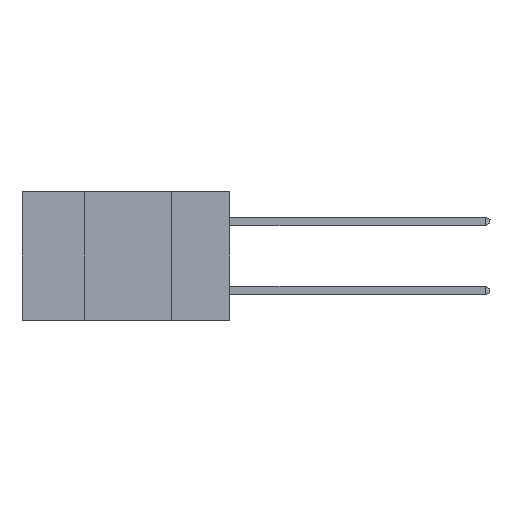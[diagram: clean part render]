
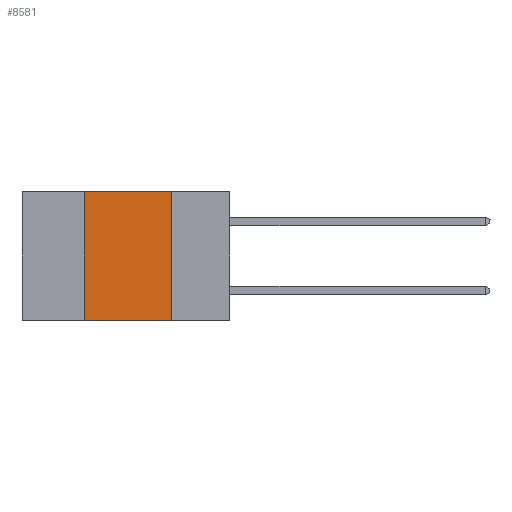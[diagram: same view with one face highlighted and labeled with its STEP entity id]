
A CAD part, left-side view. The second image highlights one B-rep face of the part: STEP entity #8581.
In plain terms, the highlighted planar face has unit normal (-1, 0, 0).
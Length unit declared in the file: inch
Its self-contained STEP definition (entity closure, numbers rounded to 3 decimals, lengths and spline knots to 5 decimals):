
#186 = ORIENTED_EDGE ( 'NONE', *, *, #3008, .F. ) ;
#297 = CARTESIAN_POINT ( 'NONE',  ( 0., 0.6, 0. ) ) ;
#744 = CARTESIAN_POINT ( 'NONE',  ( 0., 0.17, -0.37 ) ) ;
#763 = CARTESIAN_POINT ( 'NONE',  ( 0., 0.42, -0.37 ) ) ;
#1397 = VECTOR ( 'NONE', #3387, 39.37008 ) ;
#1619 = AXIS2_PLACEMENT_3D ( 'NONE', #297, #14443, #7370 ) ;
#1907 = CARTESIAN_POINT ( 'NONE',  ( 0., 0.6, 0. ) ) ;
#2742 = EDGE_CURVE ( 'NONE', #18859, #12227, #13373, .T. ) ;
#3008 = EDGE_CURVE ( 'NONE', #22088, #21772, #19269, .T. ) ;
#3387 = DIRECTION ( 'NONE',  ( 0., 0., 1. ) ) ;
#4386 = DIRECTION ( 'NONE',  ( 0., -1., 0. ) ) ;
#4478 = ORIENTED_EDGE ( 'NONE', *, *, #20597, .F. ) ;
#6117 = VECTOR ( 'NONE', #14522, 39.37008 ) ;
#7370 = DIRECTION ( 'NONE',  ( 0., 0., -1. ) ) ;
#8493 = CARTESIAN_POINT ( 'NONE',  ( 0., 0.42, -0.37 ) ) ;
#8581 = ADVANCED_FACE ( 'NONE', ( #19651 ), #16405, .F. ) ;
#9289 = EDGE_LOOP ( 'NONE', ( #18585, #4478, #186, #15371 ) ) ;
#9543 = DIRECTION ( 'NONE',  ( 0., 0., -1. ) ) ;
#10389 = CARTESIAN_POINT ( 'NONE',  ( 0., 0.42, 0. ) ) ;
#11757 = CARTESIAN_POINT ( 'NONE',  ( 0., 0.17, -0.37 ) ) ;
#12227 = VERTEX_POINT ( 'NONE', #11757 ) ;
#12552 = LINE ( 'NONE', #1907, #6117 ) ;
#12576 = CARTESIAN_POINT ( 'NONE',  ( 0., 0.17, 0. ) ) ;
#13373 = LINE ( 'NONE', #744, #20249 ) ;
#14443 = DIRECTION ( 'NONE',  ( 1., 0., 0. ) ) ;
#14522 = DIRECTION ( 'NONE',  ( 0., -1., 0. ) ) ;
#15371 = ORIENTED_EDGE ( 'NONE', *, *, #22699, .T. ) ;
#16405 = PLANE ( 'NONE',  #1619 ) ;
#18522 = LINE ( 'NONE', #19470, #19068 ) ;
#18585 = ORIENTED_EDGE ( 'NONE', *, *, #2742, .F. ) ;
#18859 = VERTEX_POINT ( 'NONE', #12576 ) ;
#19068 = VECTOR ( 'NONE', #4386, 39.37008 ) ;
#19269 = LINE ( 'NONE', #8493, #1397 ) ;
#19470 = CARTESIAN_POINT ( 'NONE',  ( 0., 0.6, -0.37 ) ) ;
#19651 = FACE_OUTER_BOUND ( 'NONE', #9289, .T. ) ;
#20249 = VECTOR ( 'NONE', #9543, 39.37008 ) ;
#20597 = EDGE_CURVE ( 'NONE', #21772, #18859, #12552, .T. ) ;
#21772 = VERTEX_POINT ( 'NONE', #10389 ) ;
#22088 = VERTEX_POINT ( 'NONE', #763 ) ;
#22699 = EDGE_CURVE ( 'NONE', #22088, #12227, #18522, .T. ) ;
